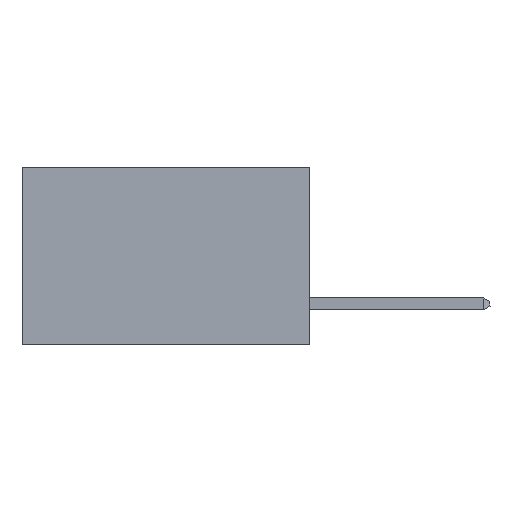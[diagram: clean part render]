
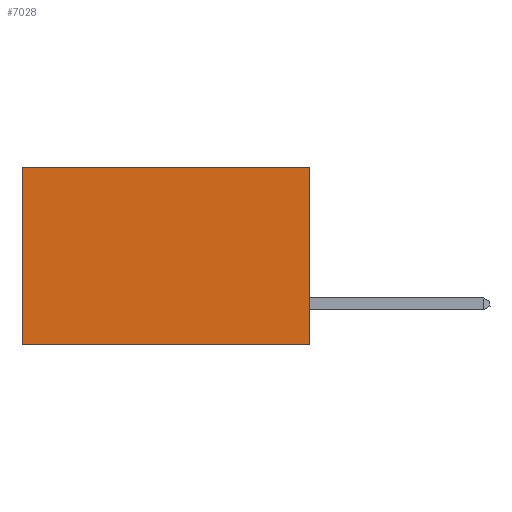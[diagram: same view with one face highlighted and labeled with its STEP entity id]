
A CAD part, left-side view. The second image highlights one B-rep face of the part: STEP entity #7028.
In plain terms, the highlighted planar face has unit normal (-1, 0, 0).
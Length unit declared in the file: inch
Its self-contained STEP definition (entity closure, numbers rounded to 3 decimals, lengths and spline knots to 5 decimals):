
#437 = LINE ( 'NONE', #11838, #5846 ) ;
#1470 = CARTESIAN_POINT ( 'NONE',  ( 0.2875, 0.6, 0. ) ) ;
#2090 = VERTEX_POINT ( 'NONE', #1470 ) ;
#2113 = LINE ( 'NONE', #6894, #10496 ) ;
#2207 = LINE ( 'NONE', #4294, #12945 ) ;
#2223 = CARTESIAN_POINT ( 'NONE',  ( 0.2875, 0., -0.37 ) ) ;
#2361 = CARTESIAN_POINT ( 'NONE',  ( 0.2875, 0., 0. ) ) ;
#3094 = EDGE_CURVE ( 'NONE', #5222, #13496, #437, .T. ) ;
#3788 = PLANE ( 'NONE',  #11905 ) ;
#3859 = CARTESIAN_POINT ( 'NONE',  ( 0.2875, 0., 0. ) ) ;
#4294 = CARTESIAN_POINT ( 'NONE',  ( 0.2875, 0.6, 0. ) ) ;
#4708 = ORIENTED_EDGE ( 'NONE', *, *, #13587, .F. ) ;
#4721 = ORIENTED_EDGE ( 'NONE', *, *, #11566, .T. ) ;
#4830 = FACE_OUTER_BOUND ( 'NONE', #8011, .T. ) ;
#4838 = ORIENTED_EDGE ( 'NONE', *, *, #12819, .T. ) ;
#4878 = ORIENTED_EDGE ( 'NONE', *, *, #3094, .F. ) ;
#5222 = VERTEX_POINT ( 'NONE', #2361 ) ;
#5427 = DIRECTION ( 'NONE',  ( 0., 0., -1. ) ) ;
#5473 = VECTOR ( 'NONE', #5794, 39.37008 ) ;
#5794 = DIRECTION ( 'NONE',  ( 0., 1., 0. ) ) ;
#5846 = VECTOR ( 'NONE', #11868, 39.37008 ) ;
#6192 = DIRECTION ( 'NONE',  ( 0., 0., -1. ) ) ;
#6894 = CARTESIAN_POINT ( 'NONE',  ( 0.2875, 0., 0. ) ) ;
#7028 = ADVANCED_FACE ( 'NONE', ( #4830 ), #3788, .F. ) ;
#7382 = CARTESIAN_POINT ( 'NONE',  ( 0.2875, 0.6, -0.37 ) ) ;
#8011 = EDGE_LOOP ( 'NONE', ( #4721, #4708, #4878, #4838 ) ) ;
#9567 = VERTEX_POINT ( 'NONE', #7382 ) ;
#10496 = VECTOR ( 'NONE', #12064, 39.37008 ) ;
#11104 = LINE ( 'NONE', #12082, #5473 ) ;
#11511 = DIRECTION ( 'NONE',  ( 1., 0., 0. ) ) ;
#11566 = EDGE_CURVE ( 'NONE', #2090, #9567, #2207, .T. ) ;
#11838 = CARTESIAN_POINT ( 'NONE',  ( 0.2875, 0., 0. ) ) ;
#11868 = DIRECTION ( 'NONE',  ( 0., 0., -1. ) ) ;
#11905 = AXIS2_PLACEMENT_3D ( 'NONE', #3859, #11511, #6192 ) ;
#12064 = DIRECTION ( 'NONE',  ( 0., 1., 0. ) ) ;
#12082 = CARTESIAN_POINT ( 'NONE',  ( 0.2875, 0., -0.37 ) ) ;
#12819 = EDGE_CURVE ( 'NONE', #5222, #2090, #2113, .T. ) ;
#12945 = VECTOR ( 'NONE', #5427, 39.37008 ) ;
#13496 = VERTEX_POINT ( 'NONE', #2223 ) ;
#13587 = EDGE_CURVE ( 'NONE', #13496, #9567, #11104, .T. ) ;
